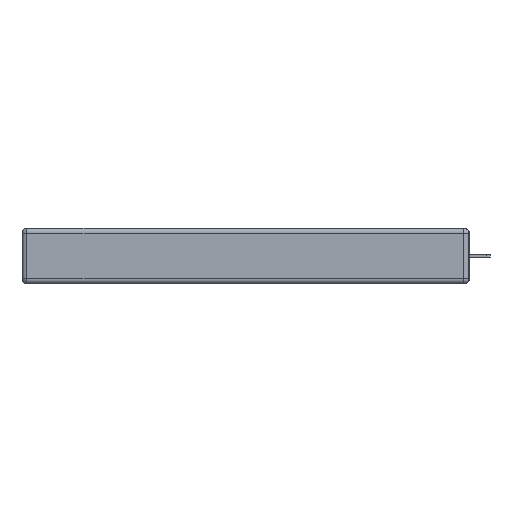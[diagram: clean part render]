
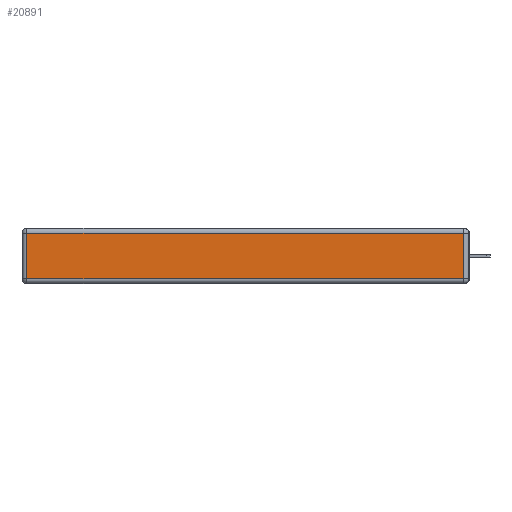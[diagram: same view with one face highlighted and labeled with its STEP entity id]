
A CAD part, left-side view. The second image highlights one B-rep face of the part: STEP entity #20891.
In plain terms, the highlighted planar face has unit normal (-1, 0, 0).
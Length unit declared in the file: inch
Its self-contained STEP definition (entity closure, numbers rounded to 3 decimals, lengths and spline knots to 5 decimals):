
#305 = EDGE_CURVE ( 'NONE', #5081, #16841, #17093, .T. ) ;
#1162 = CARTESIAN_POINT ( 'NONE',  ( 0., 0., -0.343 ) ) ;
#2371 = ORIENTED_EDGE ( 'NONE', *, *, #305, .T. ) ;
#3330 = CARTESIAN_POINT ( 'NONE',  ( 0., 2.72, -0.343 ) ) ;
#3935 = EDGE_LOOP ( 'NONE', ( #2371, #15936, #13221, #22684 ) ) ;
#4736 = DIRECTION ( 'NONE',  ( 0., -1., 0. ) ) ;
#4932 = EDGE_CURVE ( 'NONE', #7221, #5081, #5400, .T. ) ;
#5081 = VERTEX_POINT ( 'NONE', #6353 ) ;
#5400 = LINE ( 'NONE', #3330, #10565 ) ;
#5459 = DIRECTION ( 'NONE',  ( 0., 0., 1. ) ) ;
#5697 = CARTESIAN_POINT ( 'NONE',  ( 0., 0.03, -0.313 ) ) ;
#6353 = CARTESIAN_POINT ( 'NONE',  ( 0., 2.72, -0.313 ) ) ;
#6902 = LINE ( 'NONE', #17454, #26221 ) ;
#7221 = VERTEX_POINT ( 'NONE', #10856 ) ;
#8250 = VECTOR ( 'NONE', #27402, 39.37008 ) ;
#10565 = VECTOR ( 'NONE', #11802, 39.37008 ) ;
#10856 = CARTESIAN_POINT ( 'NONE',  ( 0., 2.72, -0.03 ) ) ;
#11582 = VERTEX_POINT ( 'NONE', #20227 ) ;
#11802 = DIRECTION ( 'NONE',  ( 0., 0., -1. ) ) ;
#13221 = ORIENTED_EDGE ( 'NONE', *, *, #26347, .T. ) ;
#14817 = EDGE_CURVE ( 'NONE', #16841, #11582, #16575, .T. ) ;
#15731 = PLANE ( 'NONE',  #16670 ) ;
#15936 = ORIENTED_EDGE ( 'NONE', *, *, #14817, .T. ) ;
#16575 = LINE ( 'NONE', #23084, #8250 ) ;
#16670 = AXIS2_PLACEMENT_3D ( 'NONE', #1162, #26696, #5459 ) ;
#16841 = VERTEX_POINT ( 'NONE', #5697 ) ;
#17056 = DIRECTION ( 'NONE',  ( 0., 1., 0. ) ) ;
#17093 = LINE ( 'NONE', #17634, #18809 ) ;
#17454 = CARTESIAN_POINT ( 'NONE',  ( 0., 2.75, -0.03 ) ) ;
#17634 = CARTESIAN_POINT ( 'NONE',  ( 0., 0., -0.313 ) ) ;
#18809 = VECTOR ( 'NONE', #4736, 39.37008 ) ;
#20227 = CARTESIAN_POINT ( 'NONE',  ( 0., 0.03, -0.03 ) ) ;
#20891 = ADVANCED_FACE ( 'NONE', ( #27211 ), #15731, .T. ) ;
#22684 = ORIENTED_EDGE ( 'NONE', *, *, #4932, .T. ) ;
#23084 = CARTESIAN_POINT ( 'NONE',  ( 0., 0.03, -0.343 ) ) ;
#26221 = VECTOR ( 'NONE', #17056, 39.37008 ) ;
#26347 = EDGE_CURVE ( 'NONE', #11582, #7221, #6902, .T. ) ;
#26696 = DIRECTION ( 'NONE',  ( -1., 0., 0. ) ) ;
#27211 = FACE_OUTER_BOUND ( 'NONE', #3935, .T. ) ;
#27402 = DIRECTION ( 'NONE',  ( 0., 0., 1. ) ) ;
